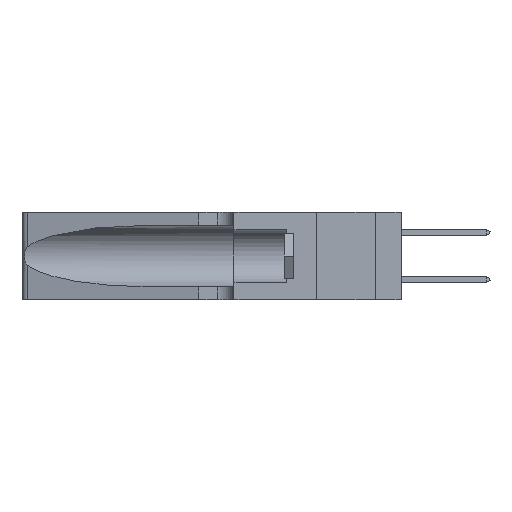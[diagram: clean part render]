
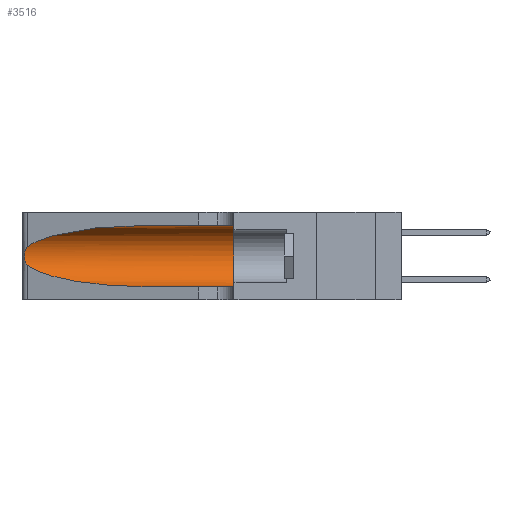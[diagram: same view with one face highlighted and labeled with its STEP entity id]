
A CAD part, left-side view. The second image highlights one B-rep face of the part: STEP entity #3516.
In plain terms, the highlighted cylindrical face has radius 3.308 mm (diameter 6.617 mm), a partial arc.
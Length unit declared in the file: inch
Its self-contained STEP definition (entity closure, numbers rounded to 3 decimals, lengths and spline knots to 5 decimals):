
#618 = CARTESIAN_POINT ( 'NONE',  ( 0.2373, 1.15595, 0.08982 ) ) ;
#1748 = EDGE_CURVE ( 'NONE', #8253, #6166, #27408, .T. ) ;
#1780 = AXIS2_PLACEMENT_3D ( 'NONE', #9879, #25058, #27185 ) ;
#1811 = AXIS2_PLACEMENT_3D ( 'NONE', #4032, #19242, #6242 ) ;
#2787 = CARTESIAN_POINT ( 'NONE',  ( 0.25487, 1.22718, 0.22369 ) ) ;
#2833 = CARTESIAN_POINT ( 'NONE',  ( 0.25487, 1.22718, 0.14631 ) ) ;
#3118 = CARTESIAN_POINT ( 'NONE',  ( 0.25787, 1.23484, 0.2124 ) ) ;
#3516 = ADVANCED_FACE ( 'NONE', ( #27191 ), #4118, .F. ) ;
#4032 = CARTESIAN_POINT ( 'NONE',  ( 0.1305, 0.35, 0.185 ) ) ;
#4118 = CYLINDRICAL_SURFACE ( 'NONE', #1780, 0.13025 ) ;
#4832 = ORIENTED_EDGE ( 'NONE', *, *, #14705, .F. ) ;
#5030 = CARTESIAN_POINT ( 'NONE',  ( 0.1305, 0.72297, 0.05475 ) ) ;
#5187 = B_SPLINE_CURVE_WITH_KNOTS ( 'NONE', 3,
 ( #22614, #13949, #16157, #3118, #18333, #5328, #20527, #7507, #22705, #9704, #24886, #11879, #27019, #14045 ),
 .UNSPECIFIED., .F., .F.,
 ( 4, 2, 2, 2, 2, 2, 4 ),
 ( 0., 0.00027, 0.00053, 0.00107, 0.0016, 0.00187, 0.00214 ),
 .UNSPECIFIED. ) ;
#5328 = CARTESIAN_POINT ( 'NONE',  ( 0.26018, 1.23835, 0.19895 ) ) ;
#5475 = CARTESIAN_POINT ( 'NONE',  ( 0.2373, 1.15595, 0.28018 ) ) ;
#6166 = VERTEX_POINT ( 'NONE', #6993 ) ;
#6221 = ORIENTED_EDGE ( 'NONE', *, *, #23844, .T. ) ;
#6242 = DIRECTION ( 'NONE',  ( 0., 0., 1. ) ) ;
#6993 = CARTESIAN_POINT ( 'NONE',  ( 0.1305, 0.72297, 0.05475 ) ) ;
#7280 =( BOUNDED_CURVE ( )  B_SPLINE_CURVE ( 3, ( #14094, #27070, #5475, #20672 ),
 .UNSPECIFIED., .F., .T. ) 
 B_SPLINE_CURVE_WITH_KNOTS ( ( 4, 4 ),
 ( 1.5708, 2.84003 ),
 .UNSPECIFIED. ) 
 CURVE ( )  GEOMETRIC_REPRESENTATION_ITEM ( )  RATIONAL_B_SPLINE_CURVE ( ( 1., 0.87, 0.87, 1. ) ) 
 REPRESENTATION_ITEM ( '' )  );
#7425 = LINE ( 'NONE', #18729, #18303 ) ;
#7507 = CARTESIAN_POINT ( 'NONE',  ( 0.26075, 1.23896, 0.178 ) ) ;
#8167 = CARTESIAN_POINT ( 'NONE',  ( 0.1305, 1.61858, 0.05475 ) ) ;
#8220 = VECTOR ( 'NONE', #23358, 39.37008 ) ;
#8253 = VERTEX_POINT ( 'NONE', #22764 ) ;
#8375 = VERTEX_POINT ( 'NONE', #10143 ) ;
#8892 = LINE ( 'NONE', #8167, #8220 ) ;
#9324 = CARTESIAN_POINT ( 'NONE',  ( 0.18966, 0.96281, 0.05475 ) ) ;
#9704 = CARTESIAN_POINT ( 'NONE',  ( 0.25856, 1.23593, 0.16098 ) ) ;
#9879 = CARTESIAN_POINT ( 'NONE',  ( 0.1305, 1.61858, 0.185 ) ) ;
#10143 = CARTESIAN_POINT ( 'NONE',  ( 0.1305, 0.72297, 0.31525 ) ) ;
#10158 = EDGE_LOOP ( 'NONE', ( #21721, #6221, #15787, #21161, #16597, #4832 ) ) ;
#10590 = EDGE_CURVE ( 'NONE', #8375, #20010, #7280, .T. ) ;
#11879 = CARTESIAN_POINT ( 'NONE',  ( 0.25639, 1.23186, 0.15144 ) ) ;
#13470 = VERTEX_POINT ( 'NONE', #14402 ) ;
#13949 = CARTESIAN_POINT ( 'NONE',  ( 0.25555, 1.22994, 0.2215 ) ) ;
#14045 = CARTESIAN_POINT ( 'NONE',  ( 0.25487, 1.22718, 0.14631 ) ) ;
#14094 = CARTESIAN_POINT ( 'NONE',  ( 0.1305, 0.72297, 0.31525 ) ) ;
#14402 = CARTESIAN_POINT ( 'NONE',  ( 0.1305, 0.35, 0.31525 ) ) ;
#14705 = EDGE_CURVE ( 'NONE', #8375, #13470, #7425, .T. ) ;
#15787 = ORIENTED_EDGE ( 'NONE', *, *, #1748, .T. ) ;
#16157 = CARTESIAN_POINT ( 'NONE',  ( 0.25639, 1.23184, 0.21858 ) ) ;
#16166 = DIRECTION ( 'NONE',  ( 0., -1., 0. ) ) ;
#16597 = ORIENTED_EDGE ( 'NONE', *, *, #18295, .F. ) ;
#18295 = EDGE_CURVE ( 'NONE', #13470, #19698, #20839, .T. ) ;
#18303 = VECTOR ( 'NONE', #16166, 39.37008 ) ;
#18333 = CARTESIAN_POINT ( 'NONE',  ( 0.25854, 1.2359, 0.20912 ) ) ;
#18729 = CARTESIAN_POINT ( 'NONE',  ( 0.1305, 1.61858, 0.31525 ) ) ;
#19242 = DIRECTION ( 'NONE',  ( 0., 1., 0. ) ) ;
#19698 = VERTEX_POINT ( 'NONE', #27913 ) ;
#20010 = VERTEX_POINT ( 'NONE', #2787 ) ;
#20527 = CARTESIAN_POINT ( 'NONE',  ( 0.26075, 1.23896, 0.19203 ) ) ;
#20672 = CARTESIAN_POINT ( 'NONE',  ( 0.25487, 1.22718, 0.22369 ) ) ;
#20839 = CIRCLE ( 'NONE', #1811, 0.13025 ) ;
#21161 = ORIENTED_EDGE ( 'NONE', *, *, #25411, .T. ) ;
#21721 = ORIENTED_EDGE ( 'NONE', *, *, #10590, .T. ) ;
#22614 = CARTESIAN_POINT ( 'NONE',  ( 0.25487, 1.22718, 0.22369 ) ) ;
#22705 = CARTESIAN_POINT ( 'NONE',  ( 0.26017, 1.23833, 0.17102 ) ) ;
#22764 = CARTESIAN_POINT ( 'NONE',  ( 0.25487, 1.22718, 0.14631 ) ) ;
#23358 = DIRECTION ( 'NONE',  ( 0., -1., 0. ) ) ;
#23844 = EDGE_CURVE ( 'NONE', #20010, #8253, #5187, .T. ) ;
#24886 = CARTESIAN_POINT ( 'NONE',  ( 0.25789, 1.23486, 0.15765 ) ) ;
#25058 = DIRECTION ( 'NONE',  ( 0., -1., 0. ) ) ;
#25411 = EDGE_CURVE ( 'NONE', #6166, #19698, #8892, .T. ) ;
#27019 = CARTESIAN_POINT ( 'NONE',  ( 0.25555, 1.22993, 0.14849 ) ) ;
#27070 = CARTESIAN_POINT ( 'NONE',  ( 0.18966, 0.96281, 0.31525 ) ) ;
#27185 = DIRECTION ( 'NONE',  ( 0., 0., -1. ) ) ;
#27191 = FACE_OUTER_BOUND ( 'NONE', #10158, .T. ) ;
#27408 =( BOUNDED_CURVE ( )  B_SPLINE_CURVE ( 3, ( #2833, #618, #9324, #5030 ),
 .UNSPECIFIED., .F., .F. ) 
 B_SPLINE_CURVE_WITH_KNOTS ( ( 4, 4 ),
 ( 3.44316, 4.71239 ),
 .UNSPECIFIED. ) 
 CURVE ( )  GEOMETRIC_REPRESENTATION_ITEM ( )  RATIONAL_B_SPLINE_CURVE ( ( 1., 0.87, 0.87, 1. ) ) 
 REPRESENTATION_ITEM ( '' )  );
#27913 = CARTESIAN_POINT ( 'NONE',  ( 0.1305, 0.35, 0.05475 ) ) ;
